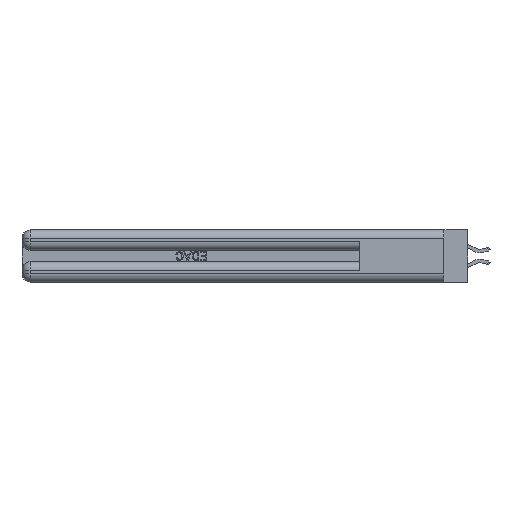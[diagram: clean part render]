
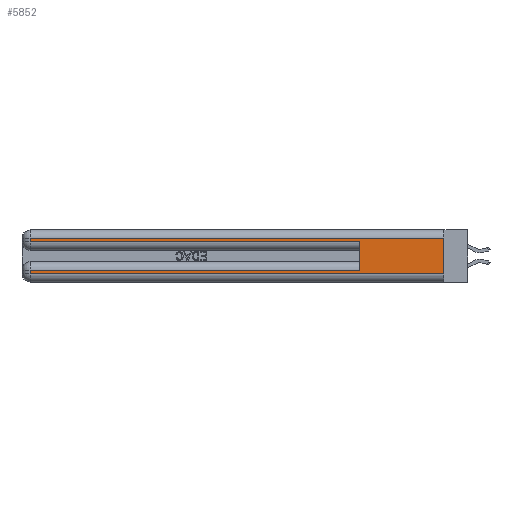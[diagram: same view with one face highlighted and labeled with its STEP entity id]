
A CAD part, left-side view. The second image highlights one B-rep face of the part: STEP entity #5852.
In plain terms, the highlighted planar face has unit normal (-1, 0, 0).
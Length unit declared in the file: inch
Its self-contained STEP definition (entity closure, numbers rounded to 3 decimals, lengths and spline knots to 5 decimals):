
#131 = LINE ( 'NONE', #41311, #13540 ) ;
#754 = CARTESIAN_POINT ( 'NONE',  ( 0., 0., 0.37 ) ) ;
#1747 = VERTEX_POINT ( 'NONE', #21901 ) ;
#2454 = CARTESIAN_POINT ( 'NONE',  ( 0., 0., 0.285 ) ) ;
#2790 = VERTEX_POINT ( 'NONE', #20261 ) ;
#3091 = CARTESIAN_POINT ( 'NONE',  ( 0., 0., 0.06 ) ) ;
#4571 = AXIS2_PLACEMENT_3D ( 'NONE', #754, #8989, #37201 ) ;
#4592 = DIRECTION ( 'NONE',  ( 0., 0., -1. ) ) ;
#4840 = CARTESIAN_POINT ( 'NONE',  ( 0., 0., 0.31 ) ) ;
#5852 = ADVANCED_FACE ( 'NONE', ( #11123 ), #25642, .F. ) ;
#6052 = LINE ( 'NONE', #13443, #19457 ) ;
#6524 = DIRECTION ( 'NONE',  ( 0., -1., 0. ) ) ;
#8989 = DIRECTION ( 'NONE',  ( 1., 0., 0. ) ) ;
#9361 = VERTEX_POINT ( 'NONE', #43659 ) ;
#9687 = EDGE_CURVE ( 'NONE', #2790, #10784, #6052, .T. ) ;
#9844 = EDGE_LOOP ( 'NONE', ( #41912, #17875, #34204, #15868, #24027, #9954, #10563, #44098 ) ) ;
#9954 = ORIENTED_EDGE ( 'NONE', *, *, #45689, .T. ) ;
#10277 = VECTOR ( 'NONE', #25305, 39.37008 ) ;
#10450 = VECTOR ( 'NONE', #6524, 39.37008 ) ;
#10563 = ORIENTED_EDGE ( 'NONE', *, *, #14267, .T. ) ;
#10784 = VERTEX_POINT ( 'NONE', #33178 ) ;
#11123 = FACE_OUTER_BOUND ( 'NONE', #9844, .T. ) ;
#12544 = LINE ( 'NONE', #36295, #10277 ) ;
#13443 = CARTESIAN_POINT ( 'NONE',  ( 0., 0., 0.37 ) ) ;
#13540 = VECTOR ( 'NONE', #27381, 39.37008 ) ;
#14267 = EDGE_CURVE ( 'NONE', #26650, #18503, #41237, .T. ) ;
#15701 = VECTOR ( 'NONE', #39211, 39.37008 ) ;
#15702 = VECTOR ( 'NONE', #37518, 39.37008 ) ;
#15868 = ORIENTED_EDGE ( 'NONE', *, *, #37520, .T. ) ;
#16067 = LINE ( 'NONE', #2454, #10450 ) ;
#16729 = CARTESIAN_POINT ( 'NONE',  ( 0., 2.94, 0.06 ) ) ;
#17379 = CARTESIAN_POINT ( 'NONE',  ( 0., 0.6, 0.285 ) ) ;
#17875 = ORIENTED_EDGE ( 'NONE', *, *, #41024, .T. ) ;
#18503 = VERTEX_POINT ( 'NONE', #16729 ) ;
#18753 = CARTESIAN_POINT ( 'NONE',  ( 0., 2.94, 0.085 ) ) ;
#19457 = VECTOR ( 'NONE', #34575, 39.37008 ) ;
#20261 = CARTESIAN_POINT ( 'NONE',  ( 0., 0., 0.31 ) ) ;
#21901 = CARTESIAN_POINT ( 'NONE',  ( 0., 0.6, 0.085 ) ) ;
#22049 = VERTEX_POINT ( 'NONE', #34227 ) ;
#23000 = LINE ( 'NONE', #3091, #15701 ) ;
#24027 = ORIENTED_EDGE ( 'NONE', *, *, #29718, .F. ) ;
#25305 = DIRECTION ( 'NONE',  ( 0., 1., 0. ) ) ;
#25642 = PLANE ( 'NONE',  #4571 ) ;
#26192 = VECTOR ( 'NONE', #26468, 39.37008 ) ;
#26468 = DIRECTION ( 'NONE',  ( 0., 0., -1. ) ) ;
#26650 = VERTEX_POINT ( 'NONE', #18753 ) ;
#27381 = DIRECTION ( 'NONE',  ( 0., 0., 1. ) ) ;
#29718 = EDGE_CURVE ( 'NONE', #1747, #42573, #131, .T. ) ;
#30675 = EDGE_CURVE ( 'NONE', #18503, #10784, #23000, .T. ) ;
#31443 = EDGE_CURVE ( 'NONE', #9361, #22049, #39200, .T. ) ;
#33178 = CARTESIAN_POINT ( 'NONE',  ( 0., 0., 0.06 ) ) ;
#34192 = LINE ( 'NONE', #4840, #15702 ) ;
#34204 = ORIENTED_EDGE ( 'NONE', *, *, #31443, .T. ) ;
#34227 = CARTESIAN_POINT ( 'NONE',  ( 0., 2.94, 0.285 ) ) ;
#34575 = DIRECTION ( 'NONE',  ( 0., 0., -1. ) ) ;
#36295 = CARTESIAN_POINT ( 'NONE',  ( 0., 0., 0.085 ) ) ;
#37201 = DIRECTION ( 'NONE',  ( 0., 0., -1. ) ) ;
#37518 = DIRECTION ( 'NONE',  ( 0., 1., 0. ) ) ;
#37520 = EDGE_CURVE ( 'NONE', #22049, #42573, #16067, .T. ) ;
#39200 = LINE ( 'NONE', #40539, #41974 ) ;
#39211 = DIRECTION ( 'NONE',  ( 0., -1., 0. ) ) ;
#40539 = CARTESIAN_POINT ( 'NONE',  ( 0., 2.94, 0.37 ) ) ;
#41024 = EDGE_CURVE ( 'NONE', #2790, #9361, #34192, .T. ) ;
#41237 = LINE ( 'NONE', #43819, #26192 ) ;
#41311 = CARTESIAN_POINT ( 'NONE',  ( 0., 0.6, 0.145 ) ) ;
#41912 = ORIENTED_EDGE ( 'NONE', *, *, #9687, .F. ) ;
#41974 = VECTOR ( 'NONE', #4592, 39.37008 ) ;
#42573 = VERTEX_POINT ( 'NONE', #17379 ) ;
#43659 = CARTESIAN_POINT ( 'NONE',  ( 0., 2.94, 0.31 ) ) ;
#43819 = CARTESIAN_POINT ( 'NONE',  ( 0., 2.94, 0.37 ) ) ;
#44098 = ORIENTED_EDGE ( 'NONE', *, *, #30675, .T. ) ;
#45689 = EDGE_CURVE ( 'NONE', #1747, #26650, #12544, .T. ) ;
